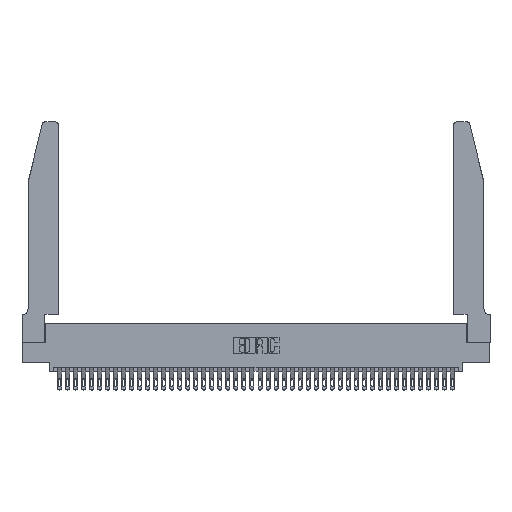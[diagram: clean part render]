
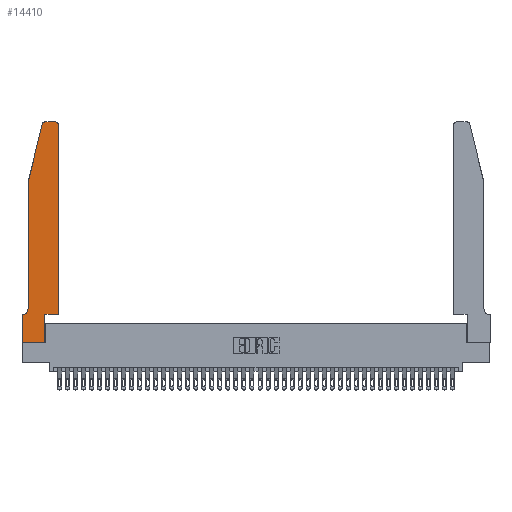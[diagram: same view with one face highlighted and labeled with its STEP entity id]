
A CAD part, top view. The second image highlights one B-rep face of the part: STEP entity #14410.
In plain terms, the highlighted planar face has unit normal (0, 0, 1).
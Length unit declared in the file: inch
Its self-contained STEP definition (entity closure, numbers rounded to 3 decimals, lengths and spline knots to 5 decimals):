
#258 = CARTESIAN_POINT ( 'NONE',  ( 0.0755, 0.42, 0.37 ) ) ;
#551 = AXIS2_PLACEMENT_3D ( 'NONE', #15403, #38554, #18802 ) ;
#1422 = VERTEX_POINT ( 'NONE', #16111 ) ;
#3400 = LINE ( 'NONE', #16363, #12563 ) ;
#3649 = CARTESIAN_POINT ( 'NONE',  ( 0.4205, 2.72, 0.37 ) ) ;
#4125 = DIRECTION ( 'NONE',  ( -1., 0., 0. ) ) ;
#4351 = LINE ( 'NONE', #38941, #12434 ) ;
#4706 = VECTOR ( 'NONE', #18547, 39.37008 ) ;
#5096 = ORIENTED_EDGE ( 'NONE', *, *, #26828, .T. ) ;
#5530 = VECTOR ( 'NONE', #32820, 39.37008 ) ;
#6137 = VECTOR ( 'NONE', #4125, 39.37008 ) ;
#6612 = LINE ( 'NONE', #12902, #5530 ) ;
#6649 = VERTEX_POINT ( 'NONE', #26937 ) ;
#7133 = DIRECTION ( 'NONE',  ( 1., 0., 0. ) ) ;
#7239 = CARTESIAN_POINT ( 'NONE',  ( 0.0755, 2., 0.37 ) ) ;
#8143 = CARTESIAN_POINT ( 'NONE',  ( 0.2865, 0., 0.37 ) ) ;
#8276 = EDGE_CURVE ( 'NONE', #20920, #40844, #17888, .T. ) ;
#8292 = LINE ( 'NONE', #21232, #6137 ) ;
#8319 = ORIENTED_EDGE ( 'NONE', *, *, #24224, .T. ) ;
#8856 = ORIENTED_EDGE ( 'NONE', *, *, #8276, .T. ) ;
#9071 = EDGE_CURVE ( 'NONE', #37317, #1422, #16227, .T. ) ;
#9136 = CARTESIAN_POINT ( 'NONE',  ( 0.0055, 0.35, 0.37 ) ) ;
#9686 = VERTEX_POINT ( 'NONE', #42137 ) ;
#9805 = VERTEX_POINT ( 'NONE', #32826 ) ;
#11525 = CARTESIAN_POINT ( 'NONE',  ( 0., 0.35, 0.37 ) ) ;
#11658 = DIRECTION ( 'NONE',  ( 1., 0., 0. ) ) ;
#11959 = CARTESIAN_POINT ( 'NONE',  ( 0.2865, 0.35, 0.37 ) ) ;
#12434 = VECTOR ( 'NONE', #22532, 39.37008 ) ;
#12563 = VECTOR ( 'NONE', #19743, 39.37008 ) ;
#12902 = CARTESIAN_POINT ( 'NONE',  ( 0.2605, 2.75, 0.37 ) ) ;
#13857 = LINE ( 'NONE', #41591, #4706 ) ;
#14410 = ADVANCED_FACE ( 'NONE', ( #32657 ), #21683, .T. ) ;
#14834 = EDGE_CURVE ( 'NONE', #31268, #33737, #24461, .T. ) ;
#15403 = CARTESIAN_POINT ( 'NONE',  ( 0.0055, 0.42, 0.37 ) ) ;
#15781 = ORIENTED_EDGE ( 'NONE', *, *, #21514, .T. ) ;
#16111 = CARTESIAN_POINT ( 'NONE',  ( 0.2865, 0.35, 0.37 ) ) ;
#16227 = LINE ( 'NONE', #11959, #34880 ) ;
#16336 = ORIENTED_EDGE ( 'NONE', *, *, #42667, .T. ) ;
#16363 = CARTESIAN_POINT ( 'NONE',  ( 0.4505, 0.35, 0.37 ) ) ;
#16839 = EDGE_CURVE ( 'NONE', #6649, #38952, #26848, .T. ) ;
#17831 = CARTESIAN_POINT ( 'NONE',  ( 0., 0., 0.37 ) ) ;
#17888 = LINE ( 'NONE', #7239, #34445 ) ;
#18343 = CARTESIAN_POINT ( 'NONE',  ( 0.284, 2.72, 0.37 ) ) ;
#18547 = DIRECTION ( 'NONE',  ( 0., 1., 0. ) ) ;
#18730 = CIRCLE ( 'NONE', #551, 0.07 ) ;
#18802 = DIRECTION ( 'NONE',  ( -1., 0., 0. ) ) ;
#18951 = ORIENTED_EDGE ( 'NONE', *, *, #42346, .T. ) ;
#19158 = EDGE_CURVE ( 'NONE', #33737, #9805, #6612, .T. ) ;
#19451 = CARTESIAN_POINT ( 'NONE',  ( 0., 0., 0.37 ) ) ;
#19743 = DIRECTION ( 'NONE',  ( 1., 0., 0. ) ) ;
#20920 = VERTEX_POINT ( 'NONE', #42288 ) ;
#21232 = CARTESIAN_POINT ( 'NONE',  ( 0.0755, 0.35, 0.37 ) ) ;
#21514 = EDGE_CURVE ( 'NONE', #32275, #20920, #4351, .T. ) ;
#21683 = PLANE ( 'NONE',  #41534 ) ;
#21690 = DIRECTION ( 'NONE',  ( 1., 0., 0. ) ) ;
#22075 = ORIENTED_EDGE ( 'NONE', *, *, #16839, .T. ) ;
#22532 = DIRECTION ( 'NONE',  ( -0.239, -0.971, 0. ) ) ;
#24067 = DIRECTION ( 'NONE',  ( 0., -1., 0. ) ) ;
#24171 = ORIENTED_EDGE ( 'NONE', *, *, #9071, .T. ) ;
#24224 = EDGE_CURVE ( 'NONE', #9686, #31268, #13857, .T. ) ;
#24461 = CIRCLE ( 'NONE', #36312, 0.03 ) ;
#25490 = EDGE_LOOP ( 'NONE', ( #39049, #32387, #15781, #8856, #26730, #18951, #22075, #5096, #24171, #16336, #8319, #27252 ) ) ;
#26730 = ORIENTED_EDGE ( 'NONE', *, *, #28215, .T. ) ;
#26828 = EDGE_CURVE ( 'NONE', #38952, #37317, #27673, .T. ) ;
#26848 = LINE ( 'NONE', #17831, #43277 ) ;
#26937 = CARTESIAN_POINT ( 'NONE',  ( 0., 0.35, 0.37 ) ) ;
#27252 = ORIENTED_EDGE ( 'NONE', *, *, #14834, .T. ) ;
#27268 = DIRECTION ( 'NONE',  ( 0., 0., 1. ) ) ;
#27673 = LINE ( 'NONE', #41092, #43069 ) ;
#28215 = EDGE_CURVE ( 'NONE', #40844, #33601, #18730, .T. ) ;
#31268 = VERTEX_POINT ( 'NONE', #42215 ) ;
#31486 = DIRECTION ( 'NONE',  ( 1., 0., 0. ) ) ;
#31637 = DIRECTION ( 'NONE',  ( 0., 0., 1. ) ) ;
#31898 = DIRECTION ( 'NONE',  ( 0., 1., 0. ) ) ;
#32275 = VERTEX_POINT ( 'NONE', #37713 ) ;
#32387 = ORIENTED_EDGE ( 'NONE', *, *, #39777, .T. ) ;
#32657 = FACE_OUTER_BOUND ( 'NONE', #25490, .T. ) ;
#32820 = DIRECTION ( 'NONE',  ( -1., 0., 0. ) ) ;
#32826 = CARTESIAN_POINT ( 'NONE',  ( 0.284, 2.75, 0.37 ) ) ;
#33601 = VERTEX_POINT ( 'NONE', #9136 ) ;
#33737 = VERTEX_POINT ( 'NONE', #36507 ) ;
#34445 = VECTOR ( 'NONE', #24067, 39.37008 ) ;
#34880 = VECTOR ( 'NONE', #31898, 39.37008 ) ;
#36312 = AXIS2_PLACEMENT_3D ( 'NONE', #3649, #27268, #7133 ) ;
#36507 = CARTESIAN_POINT ( 'NONE',  ( 0.4205, 2.75, 0.37 ) ) ;
#37317 = VERTEX_POINT ( 'NONE', #8143 ) ;
#37713 = CARTESIAN_POINT ( 'NONE',  ( 0.25487, 2.72718, 0.37 ) ) ;
#38554 = DIRECTION ( 'NONE',  ( 0., 0., -1. ) ) ;
#38941 = CARTESIAN_POINT ( 'NONE',  ( 0.0755, 2., 0.37 ) ) ;
#38952 = VERTEX_POINT ( 'NONE', #19451 ) ;
#39049 = ORIENTED_EDGE ( 'NONE', *, *, #19158, .T. ) ;
#39777 = EDGE_CURVE ( 'NONE', #9805, #32275, #42336, .T. ) ;
#40844 = VERTEX_POINT ( 'NONE', #258 ) ;
#41018 = DIRECTION ( 'NONE',  ( 0., -1., 0. ) ) ;
#41092 = CARTESIAN_POINT ( 'NONE',  ( 0., 0., 0.37 ) ) ;
#41383 = DIRECTION ( 'NONE',  ( 0., 0., 1. ) ) ;
#41534 = AXIS2_PLACEMENT_3D ( 'NONE', #11525, #31637, #11658 ) ;
#41591 = CARTESIAN_POINT ( 'NONE',  ( 0.4505, 0.35, 0.37 ) ) ;
#41838 = AXIS2_PLACEMENT_3D ( 'NONE', #18343, #41383, #21690 ) ;
#42137 = CARTESIAN_POINT ( 'NONE',  ( 0.4505, 0.35, 0.37 ) ) ;
#42215 = CARTESIAN_POINT ( 'NONE',  ( 0.4505, 2.72, 0.37 ) ) ;
#42288 = CARTESIAN_POINT ( 'NONE',  ( 0.0755, 2., 0.37 ) ) ;
#42336 = CIRCLE ( 'NONE', #41838, 0.03 ) ;
#42346 = EDGE_CURVE ( 'NONE', #33601, #6649, #8292, .T. ) ;
#42667 = EDGE_CURVE ( 'NONE', #1422, #9686, #3400, .T. ) ;
#43069 = VECTOR ( 'NONE', #31486, 39.37008 ) ;
#43277 = VECTOR ( 'NONE', #41018, 39.37008 ) ;
